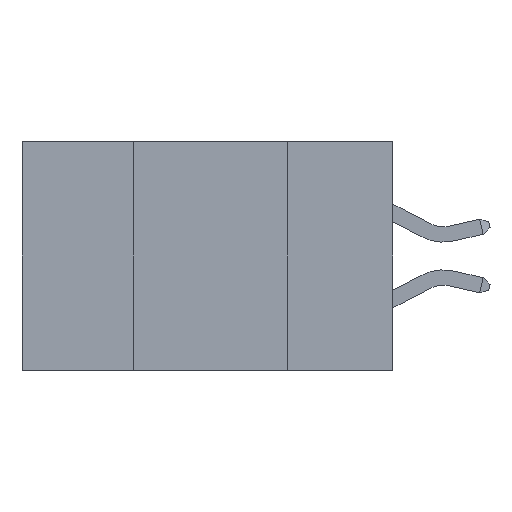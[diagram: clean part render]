
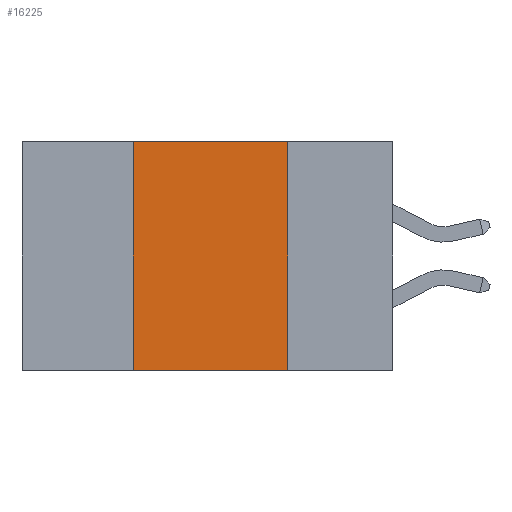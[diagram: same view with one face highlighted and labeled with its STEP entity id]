
A CAD part, left-side view. The second image highlights one B-rep face of the part: STEP entity #16225.
In plain terms, the highlighted planar face has unit normal (-1, 0, 0).
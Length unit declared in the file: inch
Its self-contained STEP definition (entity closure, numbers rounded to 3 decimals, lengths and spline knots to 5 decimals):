
#1250 = LINE ( 'NONE', #13634, #5039 ) ;
#1954 = PLANE ( 'NONE',  #11741 ) ;
#2009 = CARTESIAN_POINT ( 'NONE',  ( 0., 0.17, -0.37 ) ) ;
#2165 = VERTEX_POINT ( 'NONE', #2009 ) ;
#3058 = CARTESIAN_POINT ( 'NONE',  ( 0., 0.17, 0. ) ) ;
#3136 = CARTESIAN_POINT ( 'NONE',  ( 0., 0.6, 0. ) ) ;
#3170 = CARTESIAN_POINT ( 'NONE',  ( 0., 0.42, 0. ) ) ;
#3330 = VERTEX_POINT ( 'NONE', #3170 ) ;
#3517 = CARTESIAN_POINT ( 'NONE',  ( 0., 0.42, -0.37 ) ) ;
#3963 = LINE ( 'NONE', #3136, #17870 ) ;
#4314 = EDGE_CURVE ( 'NONE', #7817, #2165, #19464, .T. ) ;
#4959 = DIRECTION ( 'NONE',  ( 0., 0., 1. ) ) ;
#5039 = VECTOR ( 'NONE', #4959, 39.37008 ) ;
#5232 = EDGE_CURVE ( 'NONE', #8667, #3330, #1250, .T. ) ;
#5645 = DIRECTION ( 'NONE',  ( 0., 0., -1. ) ) ;
#6324 = ORIENTED_EDGE ( 'NONE', *, *, #4314, .F. ) ;
#7227 = VECTOR ( 'NONE', #21786, 39.37008 ) ;
#7365 = CARTESIAN_POINT ( 'NONE',  ( 0., 0.6, 0. ) ) ;
#7817 = VERTEX_POINT ( 'NONE', #3058 ) ;
#8290 = ORIENTED_EDGE ( 'NONE', *, *, #19027, .T. ) ;
#8667 = VERTEX_POINT ( 'NONE', #3517 ) ;
#11741 = AXIS2_PLACEMENT_3D ( 'NONE', #7365, #16021, #5645 ) ;
#12896 = EDGE_LOOP ( 'NONE', ( #6324, #16072, #19344, #8290 ) ) ;
#13634 = CARTESIAN_POINT ( 'NONE',  ( 0., 0.42, 0. ) ) ;
#13794 = VECTOR ( 'NONE', #20012, 39.37008 ) ;
#15392 = DIRECTION ( 'NONE',  ( 0., -1., 0. ) ) ;
#15475 = FACE_OUTER_BOUND ( 'NONE', #12896, .T. ) ;
#16021 = DIRECTION ( 'NONE',  ( 1., 0., 0. ) ) ;
#16072 = ORIENTED_EDGE ( 'NONE', *, *, #17198, .F. ) ;
#16225 = ADVANCED_FACE ( 'NONE', ( #15475 ), #1954, .F. ) ;
#16417 = LINE ( 'NONE', #16615, #7227 ) ;
#16615 = CARTESIAN_POINT ( 'NONE',  ( 0., 0.6, -0.37 ) ) ;
#17198 = EDGE_CURVE ( 'NONE', #3330, #7817, #3963, .T. ) ;
#17870 = VECTOR ( 'NONE', #15392, 39.37008 ) ;
#19027 = EDGE_CURVE ( 'NONE', #8667, #2165, #16417, .T. ) ;
#19344 = ORIENTED_EDGE ( 'NONE', *, *, #5232, .F. ) ;
#19464 = LINE ( 'NONE', #21768, #13794 ) ;
#20012 = DIRECTION ( 'NONE',  ( 0., 0., -1. ) ) ;
#21768 = CARTESIAN_POINT ( 'NONE',  ( 0., 0.17, 0. ) ) ;
#21786 = DIRECTION ( 'NONE',  ( 0., -1., 0. ) ) ;
